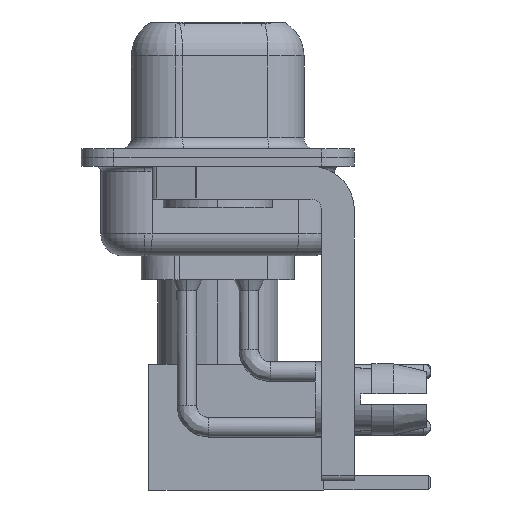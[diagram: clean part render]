
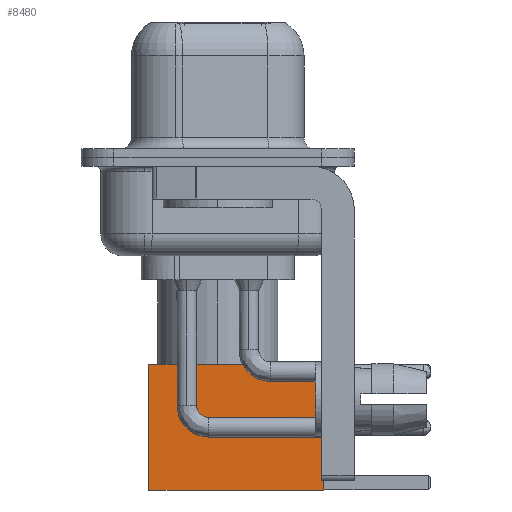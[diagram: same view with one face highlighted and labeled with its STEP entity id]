
A CAD part, left-side view. The second image highlights one B-rep face of the part: STEP entity #8480.
In plain terms, the highlighted face is planar.
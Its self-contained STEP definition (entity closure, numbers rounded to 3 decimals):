
#1095 = ORIENTED_EDGE ( 'NONE', *, *, #10219, .T. ) ;
#2166 = CARTESIAN_POINT ( 'NONE',  ( 2.875, 2.875, 8. ) ) ;
#2441 = EDGE_LOOP ( 'NONE', ( #1095, #9331, #17856, #2515 ) ) ;
#2515 = ORIENTED_EDGE ( 'NONE', *, *, #6894, .F. ) ;
#4698 = CARTESIAN_POINT ( 'NONE',  ( -2.875, 2.875, 8. ) ) ;
#4729 = VERTEX_POINT ( 'NONE', #2166 ) ;
#5265 = AXIS2_PLACEMENT_3D ( 'NONE', #9264, #18064, #14317 ) ;
#5348 = VECTOR ( 'NONE', #19573, 1000. ) ;
#5754 = LINE ( 'NONE', #20551, #11228 ) ;
#5929 = FACE_OUTER_BOUND ( 'NONE', #2441, .T. ) ;
#6708 = CARTESIAN_POINT ( 'NONE',  ( -2.875, 2.875, 0. ) ) ;
#6894 = EDGE_CURVE ( 'NONE', #4729, #11818, #8916, .T. ) ;
#7718 = EDGE_CURVE ( 'NONE', #8498, #18519, #5754, .T. ) ;
#8480 = ADVANCED_FACE ( 'NONE', ( #5929 ), #11355, .T. ) ;
#8498 = VERTEX_POINT ( 'NONE', #9930 ) ;
#8916 = LINE ( 'NONE', #15642, #17667 ) ;
#9264 = CARTESIAN_POINT ( 'NONE',  ( 2.875, 2.875, 0. ) ) ;
#9331 = ORIENTED_EDGE ( 'NONE', *, *, #7718, .T. ) ;
#9930 = CARTESIAN_POINT ( 'NONE',  ( 2.875, 2.875, 0. ) ) ;
#10219 = EDGE_CURVE ( 'NONE', #4729, #8498, #14261, .T. ) ;
#10535 = DIRECTION ( 'NONE',  ( -1., 0., 0. ) ) ;
#10696 = DIRECTION ( 'NONE',  ( -1., 0., 0. ) ) ;
#11228 = VECTOR ( 'NONE', #10535, 1000. ) ;
#11355 = PLANE ( 'NONE',  #5265 ) ;
#11818 = VERTEX_POINT ( 'NONE', #4698 ) ;
#11836 = EDGE_CURVE ( 'NONE', #11818, #18519, #21251, .T. ) ;
#12591 = DIRECTION ( 'NONE',  ( 0., 0., -1. ) ) ;
#12848 = CARTESIAN_POINT ( 'NONE',  ( -2.875, 2.875, 0. ) ) ;
#14261 = LINE ( 'NONE', #17368, #14426 ) ;
#14317 = DIRECTION ( 'NONE',  ( 0., 0., 1. ) ) ;
#14426 = VECTOR ( 'NONE', #12591, 1000. ) ;
#15642 = CARTESIAN_POINT ( 'NONE',  ( 0., 2.875, 8. ) ) ;
#17368 = CARTESIAN_POINT ( 'NONE',  ( 2.875, 2.875, 0. ) ) ;
#17667 = VECTOR ( 'NONE', #10696, 1000. ) ;
#17856 = ORIENTED_EDGE ( 'NONE', *, *, #11836, .F. ) ;
#18064 = DIRECTION ( 'NONE',  ( 0., 1., 0. ) ) ;
#18519 = VERTEX_POINT ( 'NONE', #6708 ) ;
#19573 = DIRECTION ( 'NONE',  ( 0., 0., -1. ) ) ;
#20551 = CARTESIAN_POINT ( 'NONE',  ( 0., 2.875, 0. ) ) ;
#21251 = LINE ( 'NONE', #12848, #5348 ) ;
